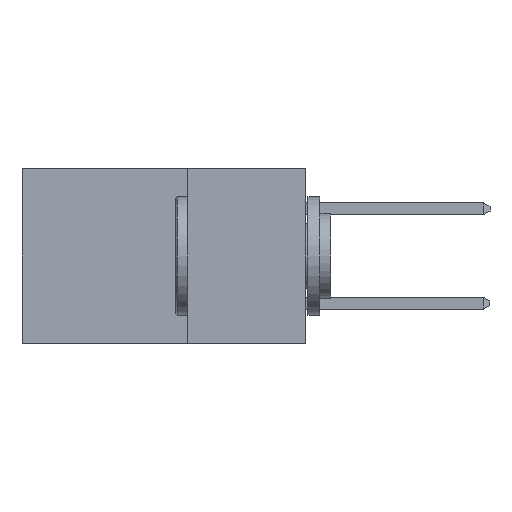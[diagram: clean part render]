
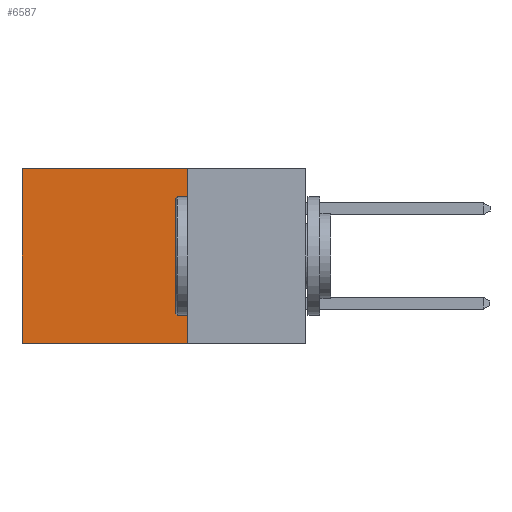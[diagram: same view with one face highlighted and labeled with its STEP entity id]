
A CAD part, left-side view. The second image highlights one B-rep face of the part: STEP entity #6587.
In plain terms, the highlighted planar face has unit normal (-1, 0, 0).
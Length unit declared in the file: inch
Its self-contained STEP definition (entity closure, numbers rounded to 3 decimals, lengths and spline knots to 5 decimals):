
#291 = VECTOR ( 'NONE', #15702, 39.37008 ) ;
#1396 = EDGE_CURVE ( 'NONE', #3098, #11970, #17547, .T. ) ;
#1442 = EDGE_LOOP ( 'NONE', ( #13386, #9411, #2561, #7417 ) ) ;
#1906 = VERTEX_POINT ( 'NONE', #3604 ) ;
#1999 = VECTOR ( 'NONE', #13666, 39.37008 ) ;
#2160 = CARTESIAN_POINT ( 'NONE',  ( 0.298, 0.25, 0. ) ) ;
#2170 = AXIS2_PLACEMENT_3D ( 'NONE', #17316, #4680, #14606 ) ;
#2561 = ORIENTED_EDGE ( 'NONE', *, *, #5548, .F. ) ;
#3098 = VERTEX_POINT ( 'NONE', #2160 ) ;
#3604 = CARTESIAN_POINT ( 'NONE',  ( 0.298, 0.25, -0.37 ) ) ;
#3884 = CARTESIAN_POINT ( 'NONE',  ( 0.298, 0.6, -0.37 ) ) ;
#4618 = LINE ( 'NONE', #8057, #291 ) ;
#4680 = DIRECTION ( 'NONE',  ( 1., 0., 0. ) ) ;
#5040 = CARTESIAN_POINT ( 'NONE',  ( 0.298, 0.6, 0. ) ) ;
#5548 = EDGE_CURVE ( 'NONE', #3098, #1906, #4618, .T. ) ;
#5911 = CARTESIAN_POINT ( 'NONE',  ( 0.298, 0.6, 0. ) ) ;
#6009 = VECTOR ( 'NONE', #15213, 39.37008 ) ;
#6393 = VECTOR ( 'NONE', #13357, 39.37008 ) ;
#6587 = ADVANCED_FACE ( 'NONE', ( #16939 ), #13206, .F. ) ;
#6786 = LINE ( 'NONE', #5040, #1999 ) ;
#6814 = CARTESIAN_POINT ( 'NONE',  ( 0.298, 0.25, -0.37 ) ) ;
#6906 = EDGE_CURVE ( 'NONE', #1906, #10035, #13961, .T. ) ;
#7417 = ORIENTED_EDGE ( 'NONE', *, *, #1396, .T. ) ;
#8057 = CARTESIAN_POINT ( 'NONE',  ( 0.298, 0.25, 0. ) ) ;
#9411 = ORIENTED_EDGE ( 'NONE', *, *, #6906, .F. ) ;
#10035 = VERTEX_POINT ( 'NONE', #3884 ) ;
#11970 = VERTEX_POINT ( 'NONE', #5911 ) ;
#13206 = PLANE ( 'NONE',  #2170 ) ;
#13357 = DIRECTION ( 'NONE',  ( 0., 1., 0. ) ) ;
#13386 = ORIENTED_EDGE ( 'NONE', *, *, #16027, .T. ) ;
#13666 = DIRECTION ( 'NONE',  ( 0., 0., -1. ) ) ;
#13961 = LINE ( 'NONE', #6814, #6009 ) ;
#14606 = DIRECTION ( 'NONE',  ( 0., 0., -1. ) ) ;
#15213 = DIRECTION ( 'NONE',  ( 0., 1., 0. ) ) ;
#15702 = DIRECTION ( 'NONE',  ( 0., 0., -1. ) ) ;
#16027 = EDGE_CURVE ( 'NONE', #11970, #10035, #6786, .T. ) ;
#16854 = CARTESIAN_POINT ( 'NONE',  ( 0.298, 0.25, 0. ) ) ;
#16939 = FACE_OUTER_BOUND ( 'NONE', #1442, .T. ) ;
#17316 = CARTESIAN_POINT ( 'NONE',  ( 0.298, 0.25, 0. ) ) ;
#17547 = LINE ( 'NONE', #16854, #6393 ) ;
